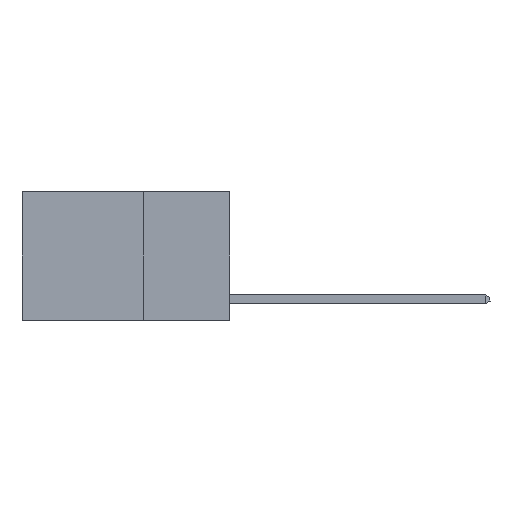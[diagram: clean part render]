
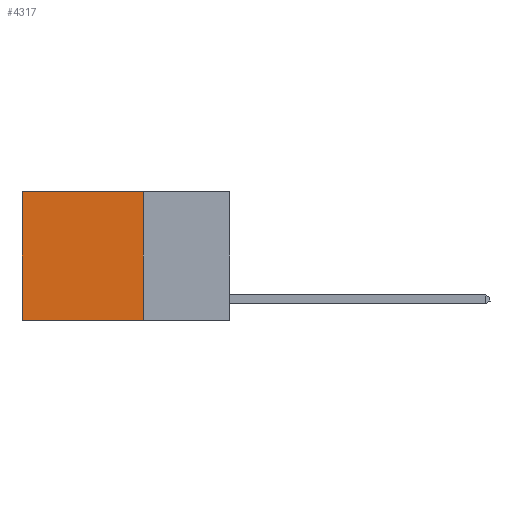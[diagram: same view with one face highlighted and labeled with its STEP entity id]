
A CAD part, left-side view. The second image highlights one B-rep face of the part: STEP entity #4317.
In plain terms, the highlighted planar face has unit normal (-1, 0, 0).
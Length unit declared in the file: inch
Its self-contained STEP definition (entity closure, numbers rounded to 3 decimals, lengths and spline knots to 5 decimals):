
#151 = EDGE_CURVE ( 'NONE', #5034, #12067, #871, .T. ) ;
#871 = LINE ( 'NONE', #22964, #12329 ) ;
#2178 = CARTESIAN_POINT ( 'NONE',  ( 0.2625, 0.25, 0. ) ) ;
#2586 = CARTESIAN_POINT ( 'NONE',  ( 0.2625, 0.25, 0. ) ) ;
#3496 = EDGE_CURVE ( 'NONE', #13867, #5034, #19631, .T. ) ;
#4186 = VECTOR ( 'NONE', #7599, 39.37008 ) ;
#4317 = ADVANCED_FACE ( 'NONE', ( #21568 ), #25475, .F. ) ;
#4388 = DIRECTION ( 'NONE',  ( 1., 0., 0. ) ) ;
#5034 = VERTEX_POINT ( 'NONE', #23582 ) ;
#5293 = CARTESIAN_POINT ( 'NONE',  ( 0.2625, 0.6, -0.37 ) ) ;
#6043 = DIRECTION ( 'NONE',  ( 0., 0., -1. ) ) ;
#6585 = ORIENTED_EDGE ( 'NONE', *, *, #151, .F. ) ;
#7286 = ORIENTED_EDGE ( 'NONE', *, *, #3496, .F. ) ;
#7347 = CARTESIAN_POINT ( 'NONE',  ( 0.2625, 0.25, 0. ) ) ;
#7599 = DIRECTION ( 'NONE',  ( 0., 0., -1. ) ) ;
#8396 = VECTOR ( 'NONE', #6043, 39.37008 ) ;
#9085 = DIRECTION ( 'NONE',  ( 0., 1., 0. ) ) ;
#10038 = VERTEX_POINT ( 'NONE', #24662 ) ;
#11371 = ORIENTED_EDGE ( 'NONE', *, *, #21401, .T. ) ;
#12067 = VERTEX_POINT ( 'NONE', #5293 ) ;
#12329 = VECTOR ( 'NONE', #25098, 39.37008 ) ;
#12692 = AXIS2_PLACEMENT_3D ( 'NONE', #2178, #4388, #19229 ) ;
#13867 = VERTEX_POINT ( 'NONE', #7347 ) ;
#15531 = LINE ( 'NONE', #24460, #4186 ) ;
#16655 = LINE ( 'NONE', #2586, #21560 ) ;
#17982 = EDGE_LOOP ( 'NONE', ( #21651, #6585, #7286, #11371 ) ) ;
#18085 = EDGE_CURVE ( 'NONE', #10038, #12067, #15531, .T. ) ;
#18726 = CARTESIAN_POINT ( 'NONE',  ( 0.2625, 0.25, 0. ) ) ;
#19229 = DIRECTION ( 'NONE',  ( 0., 0., -1. ) ) ;
#19631 = LINE ( 'NONE', #18726, #8396 ) ;
#21401 = EDGE_CURVE ( 'NONE', #13867, #10038, #16655, .T. ) ;
#21560 = VECTOR ( 'NONE', #9085, 39.37008 ) ;
#21568 = FACE_OUTER_BOUND ( 'NONE', #17982, .T. ) ;
#21651 = ORIENTED_EDGE ( 'NONE', *, *, #18085, .T. ) ;
#22964 = CARTESIAN_POINT ( 'NONE',  ( 0.2625, 0.25, -0.37 ) ) ;
#23582 = CARTESIAN_POINT ( 'NONE',  ( 0.2625, 0.25, -0.37 ) ) ;
#24460 = CARTESIAN_POINT ( 'NONE',  ( 0.2625, 0.6, 0. ) ) ;
#24662 = CARTESIAN_POINT ( 'NONE',  ( 0.2625, 0.6, 0. ) ) ;
#25098 = DIRECTION ( 'NONE',  ( 0., 1., 0. ) ) ;
#25475 = PLANE ( 'NONE',  #12692 ) ;
